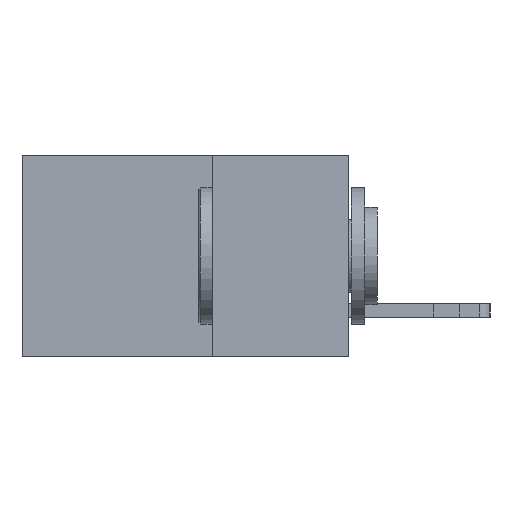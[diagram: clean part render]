
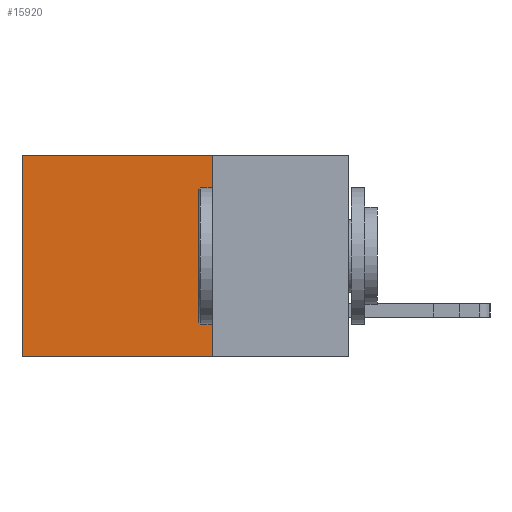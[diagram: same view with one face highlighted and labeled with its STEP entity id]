
A CAD part, left-side view. The second image highlights one B-rep face of the part: STEP entity #15920.
In plain terms, the highlighted planar face has unit normal (-1, 0, 0).
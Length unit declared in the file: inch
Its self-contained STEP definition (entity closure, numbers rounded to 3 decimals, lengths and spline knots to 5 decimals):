
#592 = DIRECTION ( 'NONE',  ( 1., 0., 0. ) ) ;
#595 = VERTEX_POINT ( 'NONE', #6104 ) ;
#1006 = VECTOR ( 'NONE', #10816, 39.37008 ) ;
#1136 = DIRECTION ( 'NONE',  ( 0., 0., -1. ) ) ;
#4851 = VECTOR ( 'NONE', #5619, 39.37008 ) ;
#5191 = LINE ( 'NONE', #5842, #1006 ) ;
#5619 = DIRECTION ( 'NONE',  ( 0., 1., 0. ) ) ;
#5842 = CARTESIAN_POINT ( 'NONE',  ( 0.298, 0.25, -0.37 ) ) ;
#6104 = CARTESIAN_POINT ( 'NONE',  ( 0.298, 0.25, 0. ) ) ;
#6868 = VECTOR ( 'NONE', #1136, 39.37008 ) ;
#6877 = PLANE ( 'NONE',  #9570 ) ;
#7117 = CARTESIAN_POINT ( 'NONE',  ( 0.298, 0.6, 0. ) ) ;
#7257 = VERTEX_POINT ( 'NONE', #11742 ) ;
#8636 = EDGE_CURVE ( 'NONE', #595, #7257, #19190, .T. ) ;
#8721 = DIRECTION ( 'NONE',  ( 0., 0., -1. ) ) ;
#8745 = ORIENTED_EDGE ( 'NONE', *, *, #8636, .F. ) ;
#9079 = CARTESIAN_POINT ( 'NONE',  ( 0.298, 0.25, 0. ) ) ;
#9139 = EDGE_CURVE ( 'NONE', #15586, #9872, #17733, .T. ) ;
#9169 = EDGE_CURVE ( 'NONE', #595, #15586, #16765, .T. ) ;
#9570 = AXIS2_PLACEMENT_3D ( 'NONE', #10074, #592, #11642 ) ;
#9575 = VECTOR ( 'NONE', #8721, 39.37008 ) ;
#9872 = VERTEX_POINT ( 'NONE', #17042 ) ;
#10074 = CARTESIAN_POINT ( 'NONE',  ( 0.298, 0.25, 0. ) ) ;
#10816 = DIRECTION ( 'NONE',  ( 0., 1., 0. ) ) ;
#11623 = EDGE_LOOP ( 'NONE', ( #18561, #17057, #8745, #12357 ) ) ;
#11642 = DIRECTION ( 'NONE',  ( 0., 0., -1. ) ) ;
#11742 = CARTESIAN_POINT ( 'NONE',  ( 0.298, 0.25, -0.37 ) ) ;
#12357 = ORIENTED_EDGE ( 'NONE', *, *, #9169, .T. ) ;
#13101 = EDGE_CURVE ( 'NONE', #7257, #9872, #5191, .T. ) ;
#14975 = CARTESIAN_POINT ( 'NONE',  ( 0.298, 0.25, 0. ) ) ;
#15340 = FACE_OUTER_BOUND ( 'NONE', #11623, .T. ) ;
#15586 = VERTEX_POINT ( 'NONE', #18442 ) ;
#15920 = ADVANCED_FACE ( 'NONE', ( #15340 ), #6877, .F. ) ;
#16765 = LINE ( 'NONE', #14975, #4851 ) ;
#17042 = CARTESIAN_POINT ( 'NONE',  ( 0.298, 0.6, -0.37 ) ) ;
#17057 = ORIENTED_EDGE ( 'NONE', *, *, #13101, .F. ) ;
#17733 = LINE ( 'NONE', #7117, #9575 ) ;
#18442 = CARTESIAN_POINT ( 'NONE',  ( 0.298, 0.6, 0. ) ) ;
#18561 = ORIENTED_EDGE ( 'NONE', *, *, #9139, .T. ) ;
#19190 = LINE ( 'NONE', #9079, #6868 ) ;
